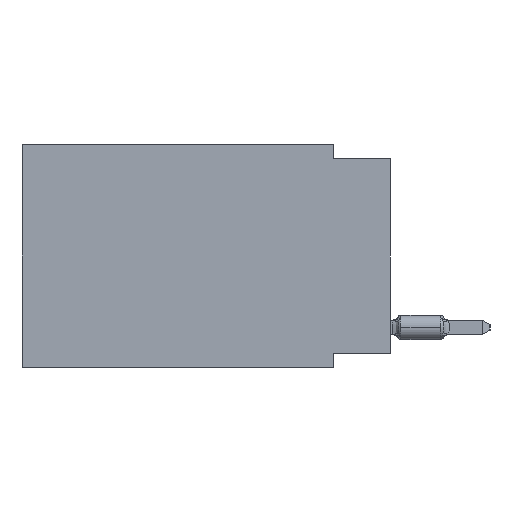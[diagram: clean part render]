
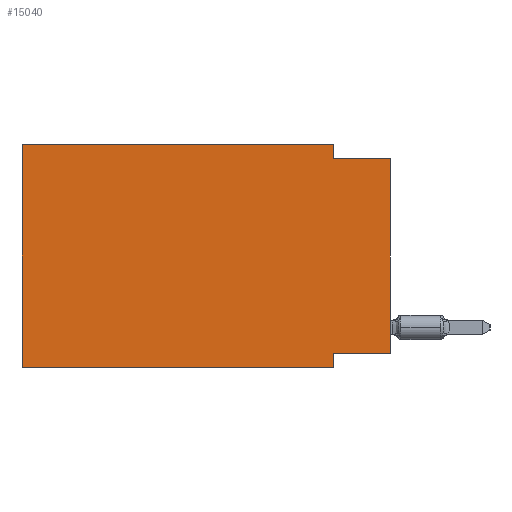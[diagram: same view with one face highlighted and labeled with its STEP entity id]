
A CAD part, left-side view. The second image highlights one B-rep face of the part: STEP entity #15040.
In plain terms, the highlighted planar face has unit normal (-1, 0, 0).
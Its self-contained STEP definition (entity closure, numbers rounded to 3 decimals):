
#79 = CARTESIAN_POINT ( 'NONE',  ( 0., 16.383, 0. ) ) ;
#81 = DIRECTION ( 'NONE',  ( 0., -1., 0. ) ) ;
#513 = CARTESIAN_POINT ( 'NONE',  ( 0., 0., -9.271 ) ) ;
#1521 = EDGE_CURVE ( 'NONE', #33911, #24024, #15251, .T. ) ;
#2995 = LINE ( 'NONE', #61371, #12216 ) ;
#3582 = AXIS2_PLACEMENT_3D ( 'NONE', #19541, #34624, #64132 ) ;
#6470 = VECTOR ( 'NONE', #20066, 1000. ) ;
#7949 = DIRECTION ( 'NONE',  ( 0., 0., 1. ) ) ;
#8020 = VECTOR ( 'NONE', #60717, 1000. ) ;
#8103 = VERTEX_POINT ( 'NONE', #32503 ) ;
#8741 = FACE_OUTER_BOUND ( 'NONE', #33635, .T. ) ;
#9915 = CARTESIAN_POINT ( 'NONE',  ( 0., 0., -0.635 ) ) ;
#12216 = VECTOR ( 'NONE', #17734, 1000. ) ;
#12451 = EDGE_CURVE ( 'NONE', #8103, #16659, #40396, .T. ) ;
#12639 = CARTESIAN_POINT ( 'NONE',  ( 0., 2.54, -0.635 ) ) ;
#15040 = ADVANCED_FACE ( 'NONE', ( #8741 ), #59840, .F. ) ;
#15251 = LINE ( 'NONE', #513, #46513 ) ;
#16573 = VECTOR ( 'NONE', #81, 1000. ) ;
#16659 = VERTEX_POINT ( 'NONE', #26678 ) ;
#16760 = VECTOR ( 'NONE', #7949, 1000. ) ;
#17225 = ORIENTED_EDGE ( 'NONE', *, *, #61835, .F. ) ;
#17734 = DIRECTION ( 'NONE',  ( 0., -1., 0. ) ) ;
#19326 = ORIENTED_EDGE ( 'NONE', *, *, #12451, .F. ) ;
#19541 = CARTESIAN_POINT ( 'NONE',  ( 0., 16.383, 0. ) ) ;
#20066 = DIRECTION ( 'NONE',  ( 0., 0., 1. ) ) ;
#20409 = CARTESIAN_POINT ( 'NONE',  ( 0., 2.54, -9.906 ) ) ;
#21221 = CARTESIAN_POINT ( 'NONE',  ( 0., 2.54, -9.906 ) ) ;
#21325 = DIRECTION ( 'NONE',  ( 0., -1., 0. ) ) ;
#21409 = CARTESIAN_POINT ( 'NONE',  ( 0., 2.54, -9.271 ) ) ;
#22919 = EDGE_CURVE ( 'NONE', #33911, #30409, #31894, .T. ) ;
#23554 = ORIENTED_EDGE ( 'NONE', *, *, #64443, .F. ) ;
#24024 = VERTEX_POINT ( 'NONE', #21409 ) ;
#25346 = CARTESIAN_POINT ( 'NONE',  ( 0., 0., -0.635 ) ) ;
#25658 = LINE ( 'NONE', #20409, #8020 ) ;
#26173 = CARTESIAN_POINT ( 'NONE',  ( 0., 2.54, 0. ) ) ;
#26678 = CARTESIAN_POINT ( 'NONE',  ( 0., 16.383, 0. ) ) ;
#29792 = ORIENTED_EDGE ( 'NONE', *, *, #22919, .T. ) ;
#30409 = VERTEX_POINT ( 'NONE', #25346 ) ;
#30804 = ORIENTED_EDGE ( 'NONE', *, *, #62030, .F. ) ;
#31894 = LINE ( 'NONE', #51881, #16760 ) ;
#32145 = CARTESIAN_POINT ( 'NONE',  ( 0., 16.383, -9.906 ) ) ;
#32503 = CARTESIAN_POINT ( 'NONE',  ( 0., 16.383, -9.906 ) ) ;
#32539 = EDGE_CURVE ( 'NONE', #43273, #58827, #46157, .T. ) ;
#33635 = EDGE_LOOP ( 'NONE', ( #29792, #23554, #44935, #30804, #19326, #55766, #17225, #39963 ) ) ;
#33911 = VERTEX_POINT ( 'NONE', #54983 ) ;
#34624 = DIRECTION ( 'NONE',  ( 1., 0., 0. ) ) ;
#35591 = DIRECTION ( 'NONE',  ( 0., 1., 0. ) ) ;
#38443 = VERTEX_POINT ( 'NONE', #21221 ) ;
#39132 = CARTESIAN_POINT ( 'NONE',  ( 0., 2.54, 0. ) ) ;
#39963 = ORIENTED_EDGE ( 'NONE', *, *, #1521, .F. ) ;
#40396 = LINE ( 'NONE', #79, #6470 ) ;
#41032 = LINE ( 'NONE', #9915, #16573 ) ;
#41245 = DIRECTION ( 'NONE',  ( 0., 0., -1. ) ) ;
#42294 = LINE ( 'NONE', #32145, #43564 ) ;
#43273 = VERTEX_POINT ( 'NONE', #39132 ) ;
#43564 = VECTOR ( 'NONE', #21325, 1000. ) ;
#44935 = ORIENTED_EDGE ( 'NONE', *, *, #32539, .F. ) ;
#46157 = LINE ( 'NONE', #26173, #53175 ) ;
#46513 = VECTOR ( 'NONE', #35591, 1000. ) ;
#49184 = EDGE_CURVE ( 'NONE', #8103, #38443, #42294, .T. ) ;
#51881 = CARTESIAN_POINT ( 'NONE',  ( 0., 0., 0. ) ) ;
#53175 = VECTOR ( 'NONE', #41245, 1000. ) ;
#54983 = CARTESIAN_POINT ( 'NONE',  ( 0., 0., -9.271 ) ) ;
#55766 = ORIENTED_EDGE ( 'NONE', *, *, #49184, .T. ) ;
#58827 = VERTEX_POINT ( 'NONE', #12639 ) ;
#59840 = PLANE ( 'NONE',  #3582 ) ;
#60717 = DIRECTION ( 'NONE',  ( 0., 0., -1. ) ) ;
#61371 = CARTESIAN_POINT ( 'NONE',  ( 0., 16.383, 0. ) ) ;
#61835 = EDGE_CURVE ( 'NONE', #24024, #38443, #25658, .T. ) ;
#62030 = EDGE_CURVE ( 'NONE', #16659, #43273, #2995, .T. ) ;
#64132 = DIRECTION ( 'NONE',  ( 0., 0., -1. ) ) ;
#64443 = EDGE_CURVE ( 'NONE', #58827, #30409, #41032, .T. ) ;
